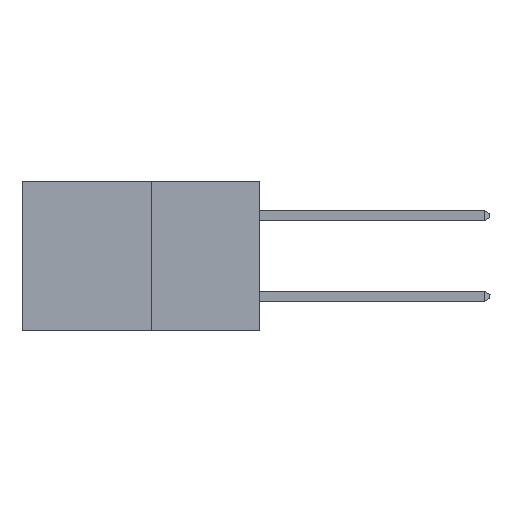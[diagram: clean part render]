
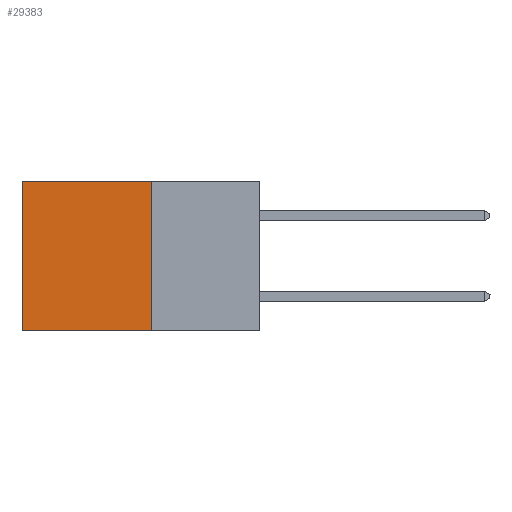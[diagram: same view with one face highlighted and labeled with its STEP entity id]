
A CAD part, left-side view. The second image highlights one B-rep face of the part: STEP entity #29383.
In plain terms, the highlighted planar face has unit normal (-1, 0, 0).
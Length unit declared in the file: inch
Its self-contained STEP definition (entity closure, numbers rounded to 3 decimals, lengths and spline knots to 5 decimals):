
#672 = CARTESIAN_POINT ( 'NONE',  ( 0.277, 0.27, -0.37 ) ) ;
#1384 = EDGE_CURVE ( 'NONE', #18951, #7721, #3894, .T. ) ;
#2011 = ORIENTED_EDGE ( 'NONE', *, *, #16006, .F. ) ;
#2182 = VECTOR ( 'NONE', #33814, 39.37008 ) ;
#3519 = CARTESIAN_POINT ( 'NONE',  ( 0.277, 0.27, 0. ) ) ;
#3848 = ORIENTED_EDGE ( 'NONE', *, *, #1384, .F. ) ;
#3894 = LINE ( 'NONE', #27453, #2182 ) ;
#6249 = CARTESIAN_POINT ( 'NONE',  ( 0.277, 0.27, -0.37 ) ) ;
#6302 = DIRECTION ( 'NONE',  ( 0., 1., 0. ) ) ;
#7413 = VECTOR ( 'NONE', #6302, 39.37008 ) ;
#7432 = CARTESIAN_POINT ( 'NONE',  ( 0.277, 0.27, -0.37 ) ) ;
#7721 = VERTEX_POINT ( 'NONE', #6249 ) ;
#8225 = VECTOR ( 'NONE', #17845, 39.37008 ) ;
#8494 = ORIENTED_EDGE ( 'NONE', *, *, #10325, .T. ) ;
#9135 = VERTEX_POINT ( 'NONE', #34272 ) ;
#10325 = EDGE_CURVE ( 'NONE', #9135, #29159, #15465, .T. ) ;
#13384 = ORIENTED_EDGE ( 'NONE', *, *, #23125, .T. ) ;
#13480 = EDGE_LOOP ( 'NONE', ( #8494, #2011, #3848, #13384 ) ) ;
#15465 = LINE ( 'NONE', #33989, #8225 ) ;
#16006 = EDGE_CURVE ( 'NONE', #7721, #29159, #25678, .T. ) ;
#16716 = CARTESIAN_POINT ( 'NONE',  ( 0.277, 0.27, 0. ) ) ;
#17076 = DIRECTION ( 'NONE',  ( 0., 1., 0. ) ) ;
#17845 = DIRECTION ( 'NONE',  ( 0., 0., -1. ) ) ;
#18371 = DIRECTION ( 'NONE',  ( 0., 0., -1. ) ) ;
#18470 = VECTOR ( 'NONE', #17076, 39.37008 ) ;
#18951 = VERTEX_POINT ( 'NONE', #16716 ) ;
#20182 = CARTESIAN_POINT ( 'NONE',  ( 0.277, 0.59, -0.37 ) ) ;
#20557 = AXIS2_PLACEMENT_3D ( 'NONE', #7432, #34517, #18371 ) ;
#23125 = EDGE_CURVE ( 'NONE', #18951, #9135, #29867, .T. ) ;
#25678 = LINE ( 'NONE', #672, #18470 ) ;
#27453 = CARTESIAN_POINT ( 'NONE',  ( 0.277, 0.27, -0.37 ) ) ;
#29159 = VERTEX_POINT ( 'NONE', #20182 ) ;
#29383 = ADVANCED_FACE ( 'NONE', ( #30459 ), #31789, .F. ) ;
#29867 = LINE ( 'NONE', #3519, #7413 ) ;
#30459 = FACE_OUTER_BOUND ( 'NONE', #13480, .T. ) ;
#31789 = PLANE ( 'NONE',  #20557 ) ;
#33814 = DIRECTION ( 'NONE',  ( 0., 0., -1. ) ) ;
#33989 = CARTESIAN_POINT ( 'NONE',  ( 0.277, 0.59, -0.37 ) ) ;
#34272 = CARTESIAN_POINT ( 'NONE',  ( 0.277, 0.59, 0. ) ) ;
#34517 = DIRECTION ( 'NONE',  ( 1., 0., 0. ) ) ;
